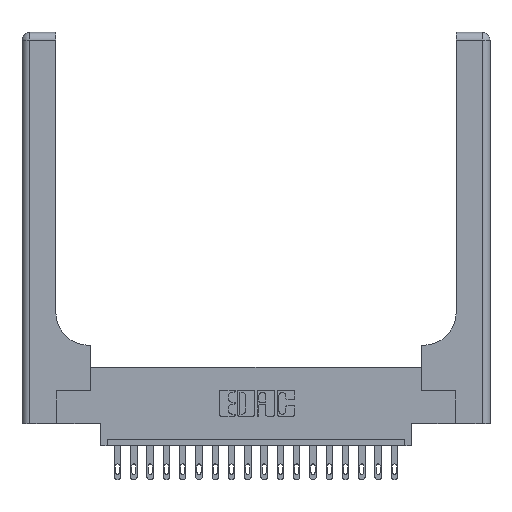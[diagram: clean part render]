
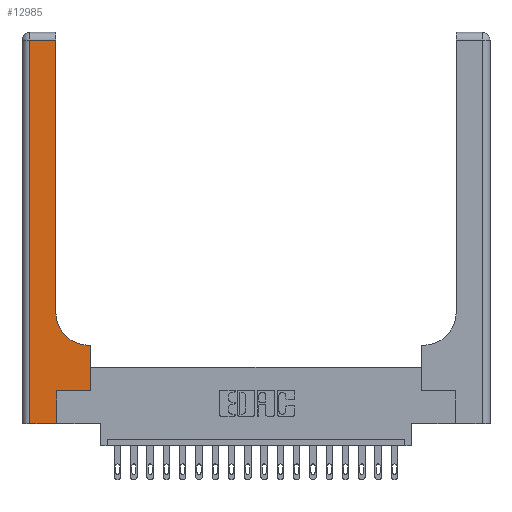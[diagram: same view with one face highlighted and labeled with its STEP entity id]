
A CAD part, top view. The second image highlights one B-rep face of the part: STEP entity #12985.
In plain terms, the highlighted planar face has unit normal (0, 0, 1).
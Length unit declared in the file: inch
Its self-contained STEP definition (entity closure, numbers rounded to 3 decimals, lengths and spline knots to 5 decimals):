
#81 = VERTEX_POINT ( 'NONE', #11410 ) ;
#485 = CARTESIAN_POINT ( 'NONE',  ( 0.26, 0.6, 0.37 ) ) ;
#673 = LINE ( 'NONE', #8390, #10132 ) ;
#721 = CARTESIAN_POINT ( 'NONE',  ( 0.528, 0.25, 0.37 ) ) ;
#1136 = CARTESIAN_POINT ( 'NONE',  ( 0.265, 0.25, 0.37 ) ) ;
#1190 = DIRECTION ( 'NONE',  ( 1., 0., 0. ) ) ;
#1774 = CARTESIAN_POINT ( 'NONE',  ( 0.26, 2.94, 0.37 ) ) ;
#1869 = AXIS2_PLACEMENT_3D ( 'NONE', #5142, #3618, #7049 ) ;
#2245 = EDGE_CURVE ( 'NONE', #7958, #7440, #14498, .T. ) ;
#2306 = CARTESIAN_POINT ( 'NONE',  ( 0.265, 0., 0.37 ) ) ;
#2496 = LINE ( 'NONE', #3906, #12309 ) ;
#2601 = VECTOR ( 'NONE', #7508, 39.37008 ) ;
#3035 = ORIENTED_EDGE ( 'NONE', *, *, #8645, .T. ) ;
#3175 = LINE ( 'NONE', #11788, #12567 ) ;
#3618 = DIRECTION ( 'NONE',  ( 0., 0., -1. ) ) ;
#3906 = CARTESIAN_POINT ( 'NONE',  ( 0., 2.94, 0.37 ) ) ;
#4001 = ORIENTED_EDGE ( 'NONE', *, *, #12687, .T. ) ;
#4183 = CARTESIAN_POINT ( 'NONE',  ( 0.26, 3., 0.37 ) ) ;
#4540 = CARTESIAN_POINT ( 'NONE',  ( 0.51, 0.85, 0.37 ) ) ;
#4627 = LINE ( 'NONE', #16894, #14244 ) ;
#5142 = CARTESIAN_POINT ( 'NONE',  ( 0., 3., 0.37 ) ) ;
#5388 = VERTEX_POINT ( 'NONE', #13361 ) ;
#6470 = VERTEX_POINT ( 'NONE', #2306 ) ;
#6478 = EDGE_CURVE ( 'NONE', #6470, #17769, #673, .T. ) ;
#7033 = CARTESIAN_POINT ( 'NONE',  ( 0.265, 0.25, 0.37 ) ) ;
#7049 = DIRECTION ( 'NONE',  ( -1., 0., 0. ) ) ;
#7440 = VERTEX_POINT ( 'NONE', #12808 ) ;
#7477 = ORIENTED_EDGE ( 'NONE', *, *, #13564, .T. ) ;
#7508 = DIRECTION ( 'NONE',  ( 1., 0., 0. ) ) ;
#7863 = DIRECTION ( 'NONE',  ( 1., 0., 0. ) ) ;
#7958 = VERTEX_POINT ( 'NONE', #14689 ) ;
#8022 = CIRCLE ( 'NONE', #15158, 0.25 ) ;
#8237 = DIRECTION ( 'NONE',  ( 0., 1., 0. ) ) ;
#8390 = CARTESIAN_POINT ( 'NONE',  ( 0.265, 0., 0.37 ) ) ;
#8491 = DIRECTION ( 'NONE',  ( 0., 1., 0. ) ) ;
#8645 = EDGE_CURVE ( 'NONE', #19446, #7958, #17675, .T. ) ;
#9024 = EDGE_LOOP ( 'NONE', ( #7477, #9339, #13183, #10879, #13551, #16816, #3035, #10441, #4001 ) ) ;
#9339 = ORIENTED_EDGE ( 'NONE', *, *, #14845, .T. ) ;
#10132 = VECTOR ( 'NONE', #8491, 39.37008 ) ;
#10441 = ORIENTED_EDGE ( 'NONE', *, *, #2245, .T. ) ;
#10879 = ORIENTED_EDGE ( 'NONE', *, *, #14548, .T. ) ;
#10971 = EDGE_CURVE ( 'NONE', #5388, #81, #3175, .T. ) ;
#11410 = CARTESIAN_POINT ( 'NONE',  ( 0.06, 0., 0.37 ) ) ;
#11788 = CARTESIAN_POINT ( 'NONE',  ( 0.06, 3., 0.37 ) ) ;
#11971 = VERTEX_POINT ( 'NONE', #16758 ) ;
#12309 = VECTOR ( 'NONE', #19919, 39.37008 ) ;
#12567 = VECTOR ( 'NONE', #16231, 39.37008 ) ;
#12687 = EDGE_CURVE ( 'NONE', #7440, #11971, #8022, .T. ) ;
#12772 = DIRECTION ( 'NONE',  ( -1., 0., 0. ) ) ;
#12808 = CARTESIAN_POINT ( 'NONE',  ( 0.51, 0.6, 0.37 ) ) ;
#12985 = ADVANCED_FACE ( 'NONE', ( #17510 ), #17715, .F. ) ;
#13183 = ORIENTED_EDGE ( 'NONE', *, *, #10971, .T. ) ;
#13303 = LINE ( 'NONE', #4183, #13570 ) ;
#13361 = CARTESIAN_POINT ( 'NONE',  ( 0.06, 2.94, 0.37 ) ) ;
#13551 = ORIENTED_EDGE ( 'NONE', *, *, #6478, .T. ) ;
#13564 = EDGE_CURVE ( 'NONE', #11971, #17224, #13303, .T. ) ;
#13570 = VECTOR ( 'NONE', #19508, 39.37008 ) ;
#14244 = VECTOR ( 'NONE', #7863, 39.37008 ) ;
#14498 = LINE ( 'NONE', #485, #16691 ) ;
#14548 = EDGE_CURVE ( 'NONE', #81, #6470, #4627, .T. ) ;
#14689 = CARTESIAN_POINT ( 'NONE',  ( 0.528, 0.6, 0.37 ) ) ;
#14795 = CARTESIAN_POINT ( 'NONE',  ( 0.528, 0.25, 0.37 ) ) ;
#14845 = EDGE_CURVE ( 'NONE', #17224, #5388, #2496, .T. ) ;
#14880 = EDGE_CURVE ( 'NONE', #17769, #19446, #19440, .T. ) ;
#15158 = AXIS2_PLACEMENT_3D ( 'NONE', #4540, #18439, #1190 ) ;
#16231 = DIRECTION ( 'NONE',  ( 0., -1., 0. ) ) ;
#16691 = VECTOR ( 'NONE', #12772, 39.37008 ) ;
#16758 = CARTESIAN_POINT ( 'NONE',  ( 0.26, 0.85, 0.37 ) ) ;
#16816 = ORIENTED_EDGE ( 'NONE', *, *, #14880, .T. ) ;
#16894 = CARTESIAN_POINT ( 'NONE',  ( 0., 0., 0.37 ) ) ;
#17030 = VECTOR ( 'NONE', #8237, 39.37008 ) ;
#17224 = VERTEX_POINT ( 'NONE', #1774 ) ;
#17510 = FACE_OUTER_BOUND ( 'NONE', #9024, .T. ) ;
#17675 = LINE ( 'NONE', #721, #17030 ) ;
#17715 = PLANE ( 'NONE',  #1869 ) ;
#17769 = VERTEX_POINT ( 'NONE', #1136 ) ;
#18439 = DIRECTION ( 'NONE',  ( 0., 0., -1. ) ) ;
#19440 = LINE ( 'NONE', #7033, #2601 ) ;
#19446 = VERTEX_POINT ( 'NONE', #14795 ) ;
#19508 = DIRECTION ( 'NONE',  ( 0., 1., 0. ) ) ;
#19919 = DIRECTION ( 'NONE',  ( -1., 0., 0. ) ) ;
